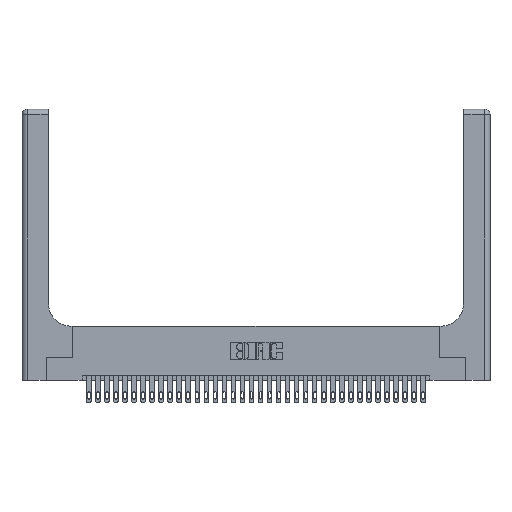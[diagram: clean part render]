
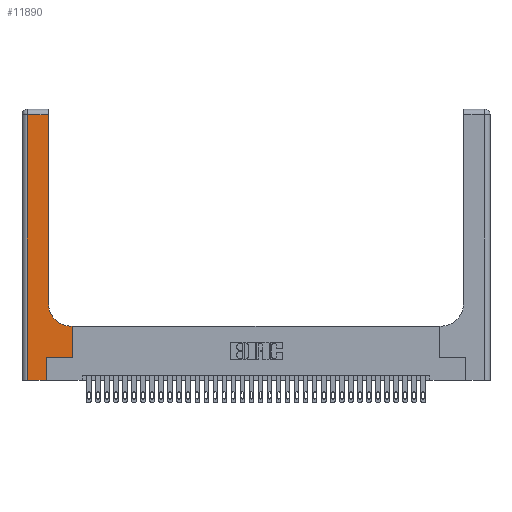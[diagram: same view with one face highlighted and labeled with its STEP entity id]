
A CAD part, top view. The second image highlights one B-rep face of the part: STEP entity #11890.
In plain terms, the highlighted planar face has unit normal (0, 0, 1).
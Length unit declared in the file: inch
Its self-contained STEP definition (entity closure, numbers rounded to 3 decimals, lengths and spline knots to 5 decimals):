
#105 = ORIENTED_EDGE ( 'NONE', *, *, #4585, .T. ) ;
#168 = EDGE_CURVE ( 'NONE', #3699, #15599, #19792, .T. ) ;
#176 = VECTOR ( 'NONE', #689, 39.37008 ) ;
#283 = LINE ( 'NONE', #24143, #33282 ) ;
#430 = CARTESIAN_POINT ( 'NONE',  ( 0.5415, 0.85, 0.37 ) ) ;
#689 = DIRECTION ( 'NONE',  ( 0., 1., 0. ) ) ;
#2068 = VERTEX_POINT ( 'NONE', #16265 ) ;
#3160 = EDGE_CURVE ( 'NONE', #15599, #2068, #283, .T. ) ;
#3526 = VERTEX_POINT ( 'NONE', #22436 ) ;
#3699 = VERTEX_POINT ( 'NONE', #21334 ) ;
#4585 = EDGE_CURVE ( 'NONE', #28886, #3526, #19852, .T. ) ;
#5323 = CARTESIAN_POINT ( 'NONE',  ( 0., 0., 0.37 ) ) ;
#5672 = DIRECTION ( 'NONE',  ( 0., 0., -1. ) ) ;
#6983 = PLANE ( 'NONE',  #31752 ) ;
#9077 = DIRECTION ( 'NONE',  ( -1., 0., 0. ) ) ;
#9447 = VECTOR ( 'NONE', #20546, 39.37008 ) ;
#10113 = ORIENTED_EDGE ( 'NONE', *, *, #168, .T. ) ;
#10222 = CARTESIAN_POINT ( 'NONE',  ( 0.269, 0.25, 0.37 ) ) ;
#11355 = VERTEX_POINT ( 'NONE', #32092 ) ;
#11890 = ADVANCED_FACE ( 'NONE', ( #22313 ), #6983, .F. ) ;
#11903 = ORIENTED_EDGE ( 'NONE', *, *, #32253, .T. ) ;
#11931 = EDGE_CURVE ( 'NONE', #13936, #30046, #30488, .T. ) ;
#11979 = DIRECTION ( 'NONE',  ( 0., 1., 0. ) ) ;
#12412 = ORIENTED_EDGE ( 'NONE', *, *, #34107, .T. ) ;
#12509 = EDGE_CURVE ( 'NONE', #11355, #13936, #17585, .T. ) ;
#13684 = DIRECTION ( 'NONE',  ( 1., 0., 0. ) ) ;
#13936 = VERTEX_POINT ( 'NONE', #27303 ) ;
#15267 = CARTESIAN_POINT ( 'NONE',  ( 0., 3., 0.37 ) ) ;
#15399 = EDGE_CURVE ( 'NONE', #3526, #18341, #21523, .T. ) ;
#15599 = VERTEX_POINT ( 'NONE', #23585 ) ;
#15632 = ORIENTED_EDGE ( 'NONE', *, *, #23936, .T. ) ;
#15920 = VECTOR ( 'NONE', #13684, 39.37008 ) ;
#16265 = CARTESIAN_POINT ( 'NONE',  ( 0.269, 0.25, 0.37 ) ) ;
#17068 = CARTESIAN_POINT ( 'NONE',  ( 0.2915, 0.85, 0.37 ) ) ;
#17585 = LINE ( 'NONE', #28656, #27012 ) ;
#17731 = CARTESIAN_POINT ( 'NONE',  ( 0.06, 2.94, 0.37 ) ) ;
#18341 = VERTEX_POINT ( 'NONE', #17731 ) ;
#19219 = DIRECTION ( 'NONE',  ( 1., 0., 0. ) ) ;
#19792 = LINE ( 'NONE', #5323, #15920 ) ;
#19852 = LINE ( 'NONE', #33507, #176 ) ;
#20162 = AXIS2_PLACEMENT_3D ( 'NONE', #430, #5672, #19219 ) ;
#20527 = VECTOR ( 'NONE', #20934, 39.37008 ) ;
#20546 = DIRECTION ( 'NONE',  ( -1., 0., 0. ) ) ;
#20934 = DIRECTION ( 'NONE',  ( 0., -1., 0. ) ) ;
#21269 = DIRECTION ( 'NONE',  ( 1., 0., 0. ) ) ;
#21334 = CARTESIAN_POINT ( 'NONE',  ( 0.06, 0., 0.37 ) ) ;
#21523 = LINE ( 'NONE', #24825, #21934 ) ;
#21934 = VECTOR ( 'NONE', #9077, 39.37008 ) ;
#22313 = FACE_OUTER_BOUND ( 'NONE', #30776, .T. ) ;
#22436 = CARTESIAN_POINT ( 'NONE',  ( 0.2915, 2.94, 0.37 ) ) ;
#23164 = CARTESIAN_POINT ( 'NONE',  ( 0.2915, 0.6, 0.37 ) ) ;
#23516 = LINE ( 'NONE', #32089, #20527 ) ;
#23585 = CARTESIAN_POINT ( 'NONE',  ( 0.269, 0., 0.37 ) ) ;
#23936 = EDGE_CURVE ( 'NONE', #18341, #3699, #23516, .T. ) ;
#24143 = CARTESIAN_POINT ( 'NONE',  ( 0.269, 0., 0.37 ) ) ;
#24825 = CARTESIAN_POINT ( 'NONE',  ( 0., 2.94, 0.37 ) ) ;
#25925 = ORIENTED_EDGE ( 'NONE', *, *, #12509, .T. ) ;
#26374 = ORIENTED_EDGE ( 'NONE', *, *, #15399, .T. ) ;
#26893 = DIRECTION ( 'NONE',  ( 0., 1., 0. ) ) ;
#27012 = VECTOR ( 'NONE', #11979, 39.37008 ) ;
#27089 = ORIENTED_EDGE ( 'NONE', *, *, #11931, .T. ) ;
#27303 = CARTESIAN_POINT ( 'NONE',  ( 0.5585, 0.6, 0.37 ) ) ;
#28656 = CARTESIAN_POINT ( 'NONE',  ( 0.5585, 0.25, 0.37 ) ) ;
#28787 = LINE ( 'NONE', #10222, #32221 ) ;
#28886 = VERTEX_POINT ( 'NONE', #17068 ) ;
#29005 = ORIENTED_EDGE ( 'NONE', *, *, #3160, .T. ) ;
#30046 = VERTEX_POINT ( 'NONE', #35225 ) ;
#30229 = CIRCLE ( 'NONE', #20162, 0.25 ) ;
#30488 = LINE ( 'NONE', #23164, #9447 ) ;
#30776 = EDGE_LOOP ( 'NONE', ( #105, #26374, #15632, #10113, #29005, #12412, #25925, #27089, #11903 ) ) ;
#31694 = DIRECTION ( 'NONE',  ( -1., 0., 0. ) ) ;
#31752 = AXIS2_PLACEMENT_3D ( 'NONE', #15267, #34100, #31694 ) ;
#32089 = CARTESIAN_POINT ( 'NONE',  ( 0.06, 3., 0.37 ) ) ;
#32092 = CARTESIAN_POINT ( 'NONE',  ( 0.5585, 0.25, 0.37 ) ) ;
#32221 = VECTOR ( 'NONE', #21269, 39.37008 ) ;
#32253 = EDGE_CURVE ( 'NONE', #30046, #28886, #30229, .T. ) ;
#33282 = VECTOR ( 'NONE', #26893, 39.37008 ) ;
#33507 = CARTESIAN_POINT ( 'NONE',  ( 0.2915, 3., 0.37 ) ) ;
#34100 = DIRECTION ( 'NONE',  ( 0., 0., -1. ) ) ;
#34107 = EDGE_CURVE ( 'NONE', #2068, #11355, #28787, .T. ) ;
#35225 = CARTESIAN_POINT ( 'NONE',  ( 0.5415, 0.6, 0.37 ) ) ;
